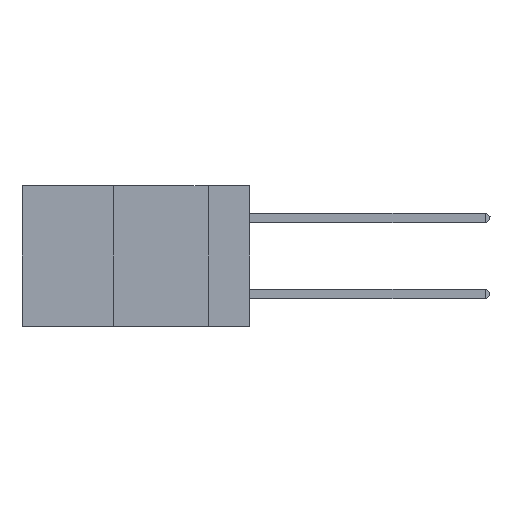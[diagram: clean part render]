
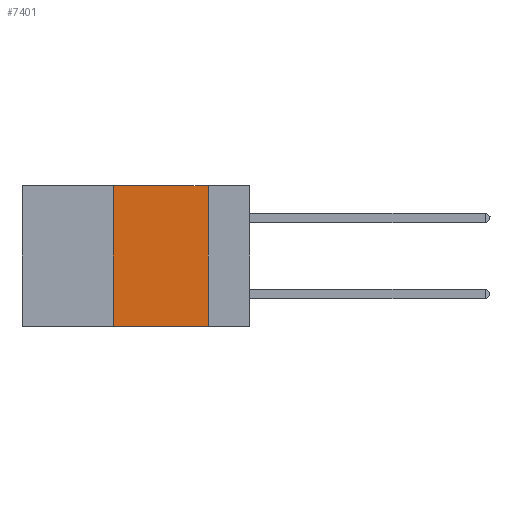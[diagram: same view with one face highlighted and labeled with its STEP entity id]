
A CAD part, left-side view. The second image highlights one B-rep face of the part: STEP entity #7401.
In plain terms, the highlighted planar face has unit normal (-1, 0, 0).
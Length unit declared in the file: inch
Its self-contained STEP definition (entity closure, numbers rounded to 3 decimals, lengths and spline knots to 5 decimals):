
#2445 = VECTOR ( 'NONE', #13662, 39.37008 ) ;
#3116 = VERTEX_POINT ( 'NONE', #14997 ) ;
#3396 = ORIENTED_EDGE ( 'NONE', *, *, #7372, .F. ) ;
#4838 = EDGE_CURVE ( 'NONE', #9848, #3116, #27485, .T. ) ;
#6047 = PLANE ( 'NONE',  #37137 ) ;
#7372 = EDGE_CURVE ( 'NONE', #3116, #37214, #23942, .T. ) ;
#7401 = ADVANCED_FACE ( 'NONE', ( #31356 ), #6047, .F. ) ;
#8998 = VERTEX_POINT ( 'NONE', #36554 ) ;
#9156 = DIRECTION ( 'NONE',  ( 0., -1., 0. ) ) ;
#9304 = DIRECTION ( 'NONE',  ( 1., 0., 0. ) ) ;
#9848 = VERTEX_POINT ( 'NONE', #11668 ) ;
#10431 = CARTESIAN_POINT ( 'NONE',  ( 0., 0.11, 0. ) ) ;
#10506 = VECTOR ( 'NONE', #16061, 39.37008 ) ;
#10536 = ORIENTED_EDGE ( 'NONE', *, *, #17756, .T. ) ;
#11083 = EDGE_LOOP ( 'NONE', ( #25987, #3396, #24578, #10536 ) ) ;
#11668 = CARTESIAN_POINT ( 'NONE',  ( 0., 0.36, -0.37 ) ) ;
#12466 = LINE ( 'NONE', #27468, #19988 ) ;
#12846 = CARTESIAN_POINT ( 'NONE',  ( 0., 0.36, 0. ) ) ;
#13662 = DIRECTION ( 'NONE',  ( 0., 0., -1. ) ) ;
#14997 = CARTESIAN_POINT ( 'NONE',  ( 0., 0.36, 0. ) ) ;
#15402 = VECTOR ( 'NONE', #9156, 39.37008 ) ;
#16061 = DIRECTION ( 'NONE',  ( 0., 0., 1. ) ) ;
#17756 = EDGE_CURVE ( 'NONE', #9848, #8998, #12466, .T. ) ;
#18688 = CARTESIAN_POINT ( 'NONE',  ( 0., 0.6, 0. ) ) ;
#19988 = VECTOR ( 'NONE', #30669, 39.37008 ) ;
#21952 = CARTESIAN_POINT ( 'NONE',  ( 0., 0.6, 0. ) ) ;
#23942 = LINE ( 'NONE', #21952, #15402 ) ;
#24578 = ORIENTED_EDGE ( 'NONE', *, *, #4838, .F. ) ;
#25987 = ORIENTED_EDGE ( 'NONE', *, *, #31305, .F. ) ;
#27468 = CARTESIAN_POINT ( 'NONE',  ( 0., 0.6, -0.37 ) ) ;
#27485 = LINE ( 'NONE', #12846, #10506 ) ;
#28047 = LINE ( 'NONE', #10431, #2445 ) ;
#30669 = DIRECTION ( 'NONE',  ( 0., -1., 0. ) ) ;
#31305 = EDGE_CURVE ( 'NONE', #37214, #8998, #28047, .T. ) ;
#31356 = FACE_OUTER_BOUND ( 'NONE', #11083, .T. ) ;
#31618 = DIRECTION ( 'NONE',  ( 0., 0., -1. ) ) ;
#36554 = CARTESIAN_POINT ( 'NONE',  ( 0., 0.11, -0.37 ) ) ;
#37137 = AXIS2_PLACEMENT_3D ( 'NONE', #18688, #9304, #31618 ) ;
#37214 = VERTEX_POINT ( 'NONE', #38385 ) ;
#38385 = CARTESIAN_POINT ( 'NONE',  ( 0., 0.11, 0. ) ) ;
